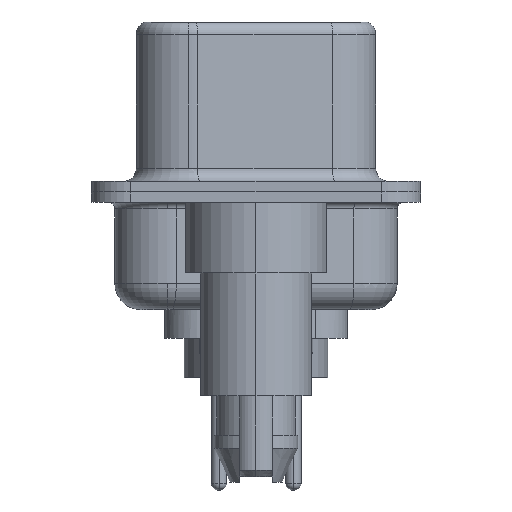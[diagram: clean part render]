
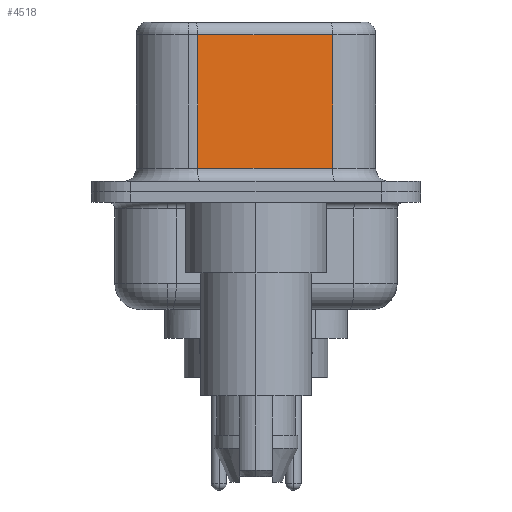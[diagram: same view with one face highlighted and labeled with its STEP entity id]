
A CAD part, left-side view. The second image highlights one B-rep face of the part: STEP entity #4518.
In plain terms, the highlighted planar face has unit normal (-0.985, -0.174, 0).
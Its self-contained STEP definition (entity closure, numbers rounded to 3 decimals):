
#94 = LINE ( 'NONE', #3285, #6636 ) ;
#514 = CARTESIAN_POINT ( 'NONE',  ( 4.58, -2.927, 6.52 ) ) ;
#661 = LINE ( 'NONE', #2279, #6118 ) ;
#760 = CARTESIAN_POINT ( 'NONE',  ( 3.67, 2.233, 0.9 ) ) ;
#949 = CARTESIAN_POINT ( 'NONE',  ( 4.58, -2.927, 0.9 ) ) ;
#2132 = EDGE_CURVE ( 'NONE', #13439, #9425, #94, .T. ) ;
#2279 = CARTESIAN_POINT ( 'NONE',  ( 3.67, 2.233, 6.52 ) ) ;
#2600 = VECTOR ( 'NONE', #12146, 1000. ) ;
#3285 = CARTESIAN_POINT ( 'NONE',  ( 4.58, -2.927, 0.9 ) ) ;
#3418 = VECTOR ( 'NONE', #5093, 1000. ) ;
#4106 = ORIENTED_EDGE ( 'NONE', *, *, #8832, .T. ) ;
#4518 = ADVANCED_FACE ( 'NONE', ( #8954 ), #10728, .F. ) ;
#4586 = DIRECTION ( 'NONE',  ( 0., 0., -1. ) ) ;
#4949 = ORIENTED_EDGE ( 'NONE', *, *, #2132, .T. ) ;
#5093 = DIRECTION ( 'NONE',  ( -0.174, 0.985, 0. ) ) ;
#5962 = VERTEX_POINT ( 'NONE', #11375 ) ;
#6118 = VECTOR ( 'NONE', #4586, 1000. ) ;
#6636 = VECTOR ( 'NONE', #11509, 1000. ) ;
#7557 = CARTESIAN_POINT ( 'NONE',  ( 4.58, -2.927, 6.52 ) ) ;
#8494 = VERTEX_POINT ( 'NONE', #12977 ) ;
#8832 = EDGE_CURVE ( 'NONE', #5962, #13439, #661, .T. ) ;
#8954 = FACE_OUTER_BOUND ( 'NONE', #11359, .T. ) ;
#9425 = VERTEX_POINT ( 'NONE', #949 ) ;
#9471 = DIRECTION ( 'NONE',  ( -0.174, 0.985, 0. ) ) ;
#10116 = DIRECTION ( 'NONE',  ( 0.985, 0.174, 0. ) ) ;
#10728 = PLANE ( 'NONE',  #12499 ) ;
#11217 = EDGE_CURVE ( 'NONE', #8494, #9425, #11883, .T. ) ;
#11359 = EDGE_LOOP ( 'NONE', ( #12635, #11986, #4106, #4949 ) ) ;
#11375 = CARTESIAN_POINT ( 'NONE',  ( 3.67, 2.233, 6.02 ) ) ;
#11509 = DIRECTION ( 'NONE',  ( 0.174, -0.985, 0. ) ) ;
#11883 = LINE ( 'NONE', #514, #2600 ) ;
#11986 = ORIENTED_EDGE ( 'NONE', *, *, #14828, .T. ) ;
#12146 = DIRECTION ( 'NONE',  ( 0., 0., -1. ) ) ;
#12314 = LINE ( 'NONE', #13167, #3418 ) ;
#12499 = AXIS2_PLACEMENT_3D ( 'NONE', #7557, #10116, #9471 ) ;
#12635 = ORIENTED_EDGE ( 'NONE', *, *, #11217, .F. ) ;
#12977 = CARTESIAN_POINT ( 'NONE',  ( 4.58, -2.927, 6.02 ) ) ;
#13167 = CARTESIAN_POINT ( 'NONE',  ( 4.58, -2.927, 6.02 ) ) ;
#13439 = VERTEX_POINT ( 'NONE', #760 ) ;
#14828 = EDGE_CURVE ( 'NONE', #8494, #5962, #12314, .T. ) ;
